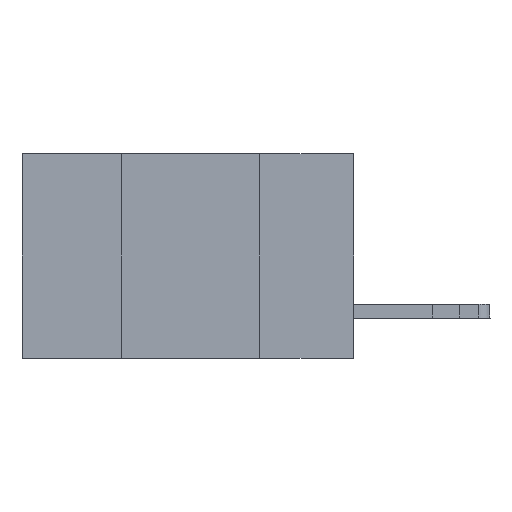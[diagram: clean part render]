
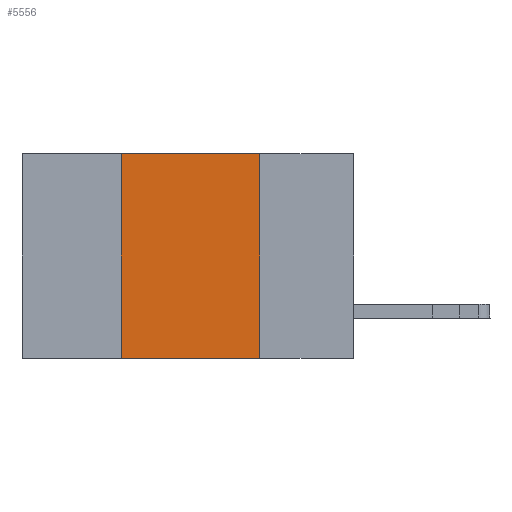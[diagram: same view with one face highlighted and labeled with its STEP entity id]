
A CAD part, left-side view. The second image highlights one B-rep face of the part: STEP entity #5556.
In plain terms, the highlighted planar face has unit normal (-1, 0, 0).
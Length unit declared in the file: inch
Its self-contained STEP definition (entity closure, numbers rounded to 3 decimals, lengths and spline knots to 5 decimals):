
#258 = CARTESIAN_POINT ( 'NONE',  ( 0., 0.42, 0. ) ) ;
#585 = LINE ( 'NONE', #5406, #3755 ) ;
#1779 = AXIS2_PLACEMENT_3D ( 'NONE', #4612, #15858, #7681 ) ;
#2022 = ORIENTED_EDGE ( 'NONE', *, *, #5547, .F. ) ;
#2037 = ORIENTED_EDGE ( 'NONE', *, *, #7818, .T. ) ;
#2485 = EDGE_LOOP ( 'NONE', ( #5953, #2022, #10718, #2037 ) ) ;
#3397 = DIRECTION ( 'NONE',  ( 0., -1., 0. ) ) ;
#3409 = CARTESIAN_POINT ( 'NONE',  ( 0., 0.42, 0. ) ) ;
#3755 = VECTOR ( 'NONE', #10472, 39.37008 ) ;
#4043 = CARTESIAN_POINT ( 'NONE',  ( 0., 0.17, 0. ) ) ;
#4612 = CARTESIAN_POINT ( 'NONE',  ( 0., 0.6, 0. ) ) ;
#4690 = CARTESIAN_POINT ( 'NONE',  ( 0., 0.17, -0.37 ) ) ;
#5406 = CARTESIAN_POINT ( 'NONE',  ( 0., 0.6, 0. ) ) ;
#5547 = EDGE_CURVE ( 'NONE', #12497, #13373, #585, .T. ) ;
#5556 = ADVANCED_FACE ( 'NONE', ( #10191 ), #16205, .F. ) ;
#5953 = ORIENTED_EDGE ( 'NONE', *, *, #13565, .F. ) ;
#6337 = VERTEX_POINT ( 'NONE', #4690 ) ;
#6913 = VERTEX_POINT ( 'NONE', #15515 ) ;
#7681 = DIRECTION ( 'NONE',  ( 0., 0., -1. ) ) ;
#7818 = EDGE_CURVE ( 'NONE', #6913, #6337, #13929, .T. ) ;
#9461 = DIRECTION ( 'NONE',  ( 0., 0., -1. ) ) ;
#9831 = CARTESIAN_POINT ( 'NONE',  ( 0., 0.6, -0.37 ) ) ;
#10191 = FACE_OUTER_BOUND ( 'NONE', #2485, .T. ) ;
#10472 = DIRECTION ( 'NONE',  ( 0., -1., 0. ) ) ;
#10718 = ORIENTED_EDGE ( 'NONE', *, *, #11991, .F. ) ;
#10721 = VECTOR ( 'NONE', #3397, 39.37008 ) ;
#11001 = LINE ( 'NONE', #3409, #13800 ) ;
#11176 = DIRECTION ( 'NONE',  ( 0., 0., 1. ) ) ;
#11411 = VECTOR ( 'NONE', #9461, 39.37008 ) ;
#11991 = EDGE_CURVE ( 'NONE', #6913, #12497, #11001, .T. ) ;
#12002 = CARTESIAN_POINT ( 'NONE',  ( 0., 0.17, 0. ) ) ;
#12497 = VERTEX_POINT ( 'NONE', #258 ) ;
#13373 = VERTEX_POINT ( 'NONE', #4043 ) ;
#13565 = EDGE_CURVE ( 'NONE', #13373, #6337, #14153, .T. ) ;
#13800 = VECTOR ( 'NONE', #11176, 39.37008 ) ;
#13929 = LINE ( 'NONE', #9831, #10721 ) ;
#14153 = LINE ( 'NONE', #12002, #11411 ) ;
#15515 = CARTESIAN_POINT ( 'NONE',  ( 0., 0.42, -0.37 ) ) ;
#15858 = DIRECTION ( 'NONE',  ( 1., 0., 0. ) ) ;
#16205 = PLANE ( 'NONE',  #1779 ) ;
